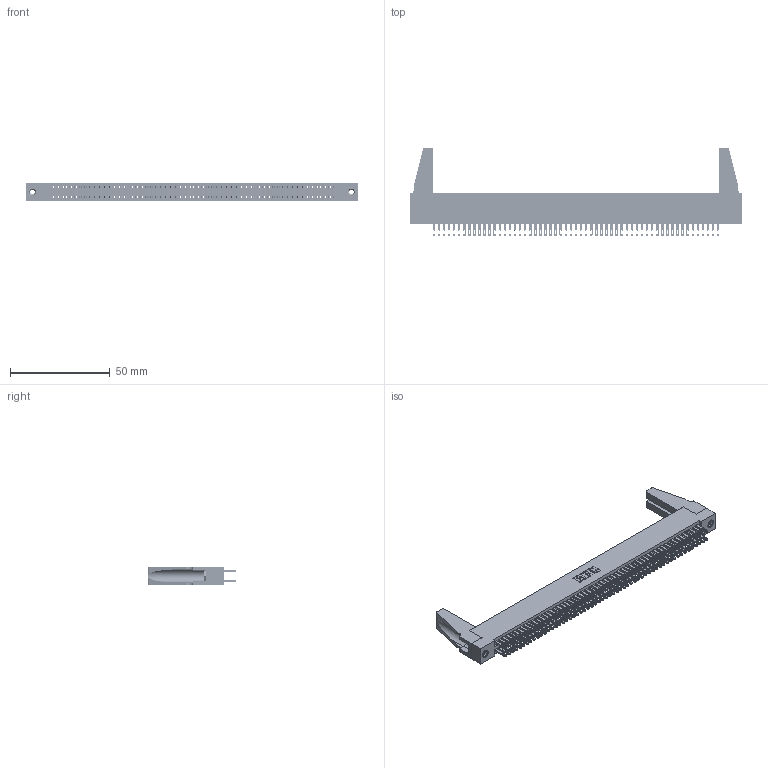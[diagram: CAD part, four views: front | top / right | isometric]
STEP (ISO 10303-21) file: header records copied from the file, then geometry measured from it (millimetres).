
FILE_DESCRIPTION (( 'STEP AP203' ), '1' );
FILE_NAME ('345-114-500-288.STEP', '2019-11-05T00:32:11', ( '' ), ( '' ), 'SwSTEP 2.0', 'SolidWorks 2016', '' );
FILE_SCHEMA (( 'CONFIG_CONTROL_DESIGN' ));
Length unit declared in the file: inch
Products named in the file (5): 345-114-500-288; 345 Part_Flush Mounting Lugs - 0.156 Dia-TH; 345-220-078_345-220-088; 345-292-001_345-293-100; 345-250-001_345-250-001-102
Assembly tree (119 placements, depth 2):
  345-114-500-288
    345 Part_Flush Mounting Lugs - 0.156 Dia-TH
    345-292-001_345-293-100  x114
    345-250-001_345-250-001-102  x2
    345-220-078_345-220-088  x2
Bounding box: 166.01 x 44.37 x 9.4 mm (x, y, z)
Volume: 19866.9 mm3; surface area: 29134.3 mm2
Topology: 119 solids, 119 shells, 5494 faces, 16729 edges, 11142 vertices
Faces by surface type: plane 3230, cylinder 2248, cone 12, torus 4
Entity records: 44782 total; most frequent: CARTESIAN_POINT 7486, ORIENTED_EDGE 7380, DIRECTION 6590, EDGE_CURVE 3690, LINE 3284, VECTOR 3284, VERTEX_POINT 2454, AXIS2_PLACEMENT_3D 1653
